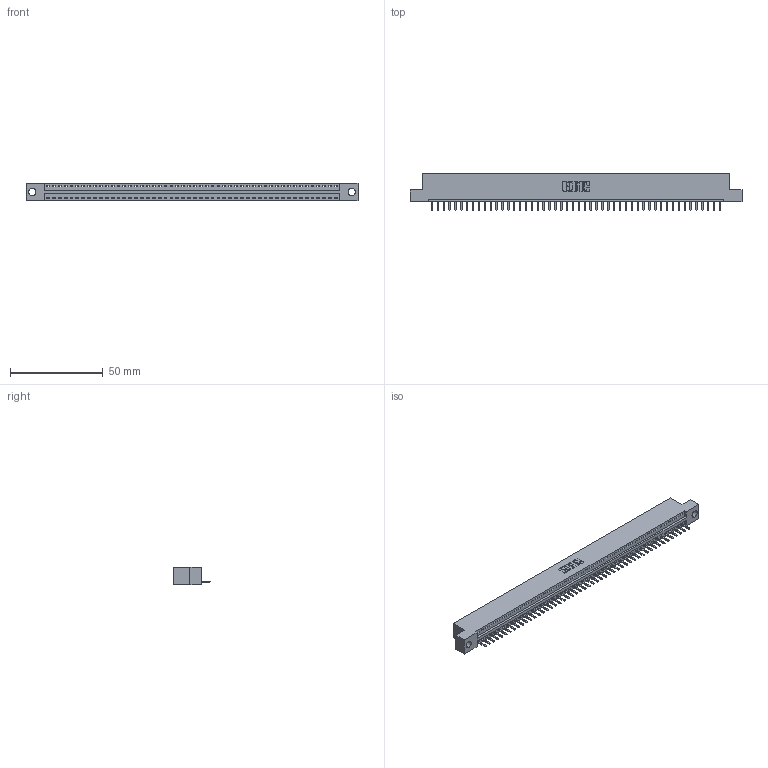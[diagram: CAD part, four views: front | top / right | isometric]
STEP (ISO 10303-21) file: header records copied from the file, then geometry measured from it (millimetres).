
FILE_DESCRIPTION (( 'STEP AP203' ), '1' );
FILE_NAME ('346-050-520-104.STEP', '2018-08-25T13:14:34', ( '' ), ( '' ), 'SwSTEP 2.0', 'SolidWorks 2016', '' );
FILE_SCHEMA (( 'CONFIG_CONTROL_DESIGN' ));
Length unit declared in the file: inch
Products named in the file (3): 346-050-520-104; 346 Part_Flush Mounting Lugs - 0.156 Dia-TH; 345-292-001_345-293-120
Assembly tree (51 placements, depth 2):
  346-050-520-104
    346 Part_Flush Mounting Lugs - 0.156 Dia-TH
    345-292-001_345-293-120  x50
Bounding box: 179.32 x 20.02 x 9.4 mm (x, y, z)
Volume: 16988.7 mm3; surface area: 20644.9 mm2
Topology: 51 solids, 51 shells, 3222 faces, 9529 edges, 6218 vertices
Faces by surface type: plane 2176, cylinder 1046
Entity records: 30071 total; most frequent: CARTESIAN_POINT 5170, ORIENTED_EDGE 5142, DIRECTION 4539, EDGE_CURVE 2571, VECTOR 2235, LINE 2235, VERTEX_POINT 1710, AXIS2_PLACEMENT_3D 1152
